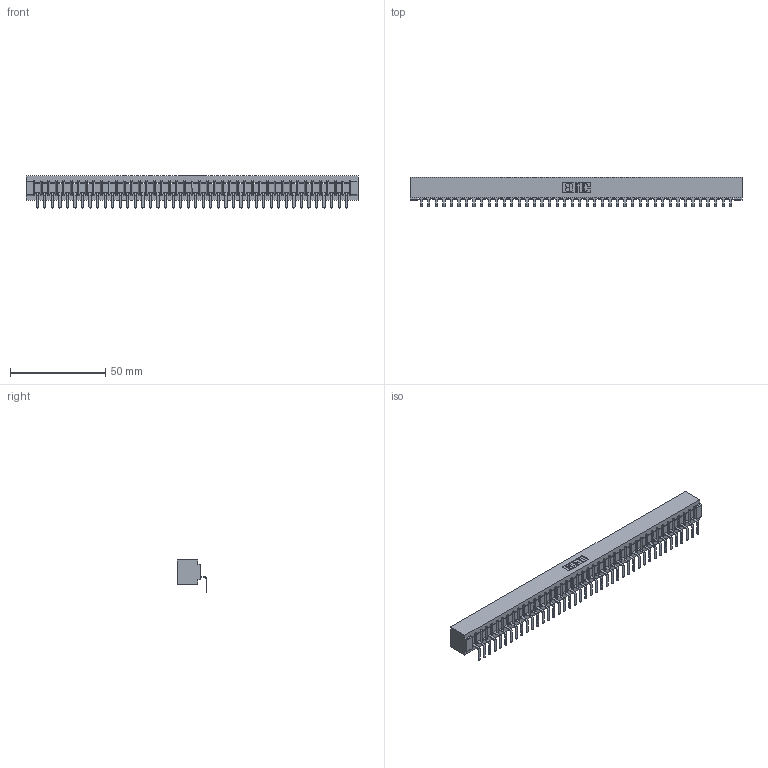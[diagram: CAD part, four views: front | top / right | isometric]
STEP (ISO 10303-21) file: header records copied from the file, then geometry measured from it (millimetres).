
FILE_DESCRIPTION (( 'STEP AP203' ), '1' );
FILE_NAME ('307-042-559-101.STEP', '2019-09-05T17:20:21', ( '' ), ( '' ), 'SwSTEP 2.0', 'SolidWorks 2016', '' );
FILE_SCHEMA (( 'CONFIG_CONTROL_DESIGN' ));
Length unit declared in the file: inch
Products named in the file (3): 307 Part_No Mounting Lugs; 307-042-559-101; 307-290-001_558 559 - 1 (Single)
Assembly tree (43 placements, depth 2):
  307-042-559-101
    307 Part_No Mounting Lugs
    307-290-001_558 559 - 1 (Single)  x42
Bounding box: 174.29 x 15.46 x 16.8 mm (x, y, z)
Volume: 18654.6 mm3; surface area: 20198.4 mm2
Topology: 43 solids, 43 shells, 2673 faces, 7607 edges, 4898 vertices
Faces by surface type: plane 1704, cylinder 883, sphere 86
Entity records: 35832 total; most frequent: CARTESIAN_POINT 6036, ORIENTED_EDGE 6022, DIRECTION 5869, EDGE_CURVE 3011, LINE 2311, VECTOR 2311, VERTEX_POINT 1946, AXIS2_PLACEMENT_3D 1779
